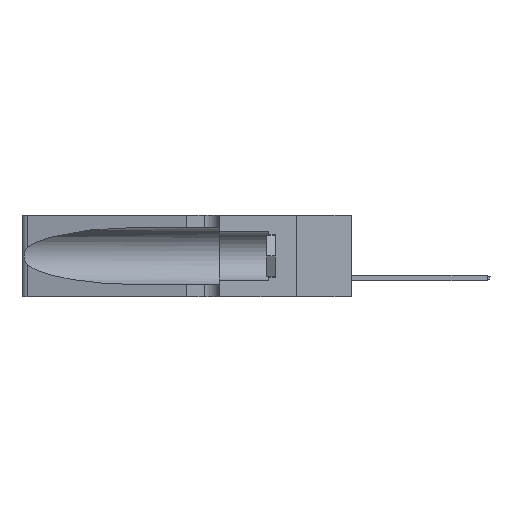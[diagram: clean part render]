
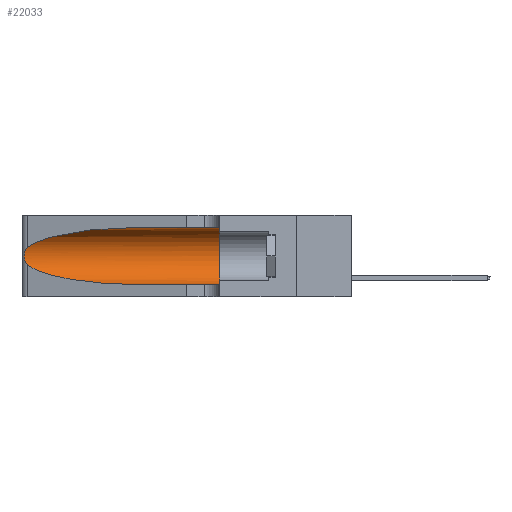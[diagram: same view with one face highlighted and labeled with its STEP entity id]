
A CAD part, left-side view. The second image highlights one B-rep face of the part: STEP entity #22033.
In plain terms, the highlighted cylindrical face has radius 3.308 mm (diameter 6.617 mm), a partial arc.
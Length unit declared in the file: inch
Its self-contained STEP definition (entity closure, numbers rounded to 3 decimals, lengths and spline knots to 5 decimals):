
#607 = LINE ( 'NONE', #9690, #24360 ) ;
#701 = AXIS2_PLACEMENT_3D ( 'NONE', #26707, #38250, #37762 ) ;
#719 = VERTEX_POINT ( 'NONE', #9431 ) ;
#1032 = CARTESIAN_POINT ( 'NONE',  ( 0.25487, 1.22718, 0.14631 ) ) ;
#1111 = CARTESIAN_POINT ( 'NONE',  ( 0.26075, 1.23896, 0.19203 ) ) ;
#1333 = EDGE_CURVE ( 'NONE', #11375, #21512, #15823, .T. ) ;
#2590 = ORIENTED_EDGE ( 'NONE', *, *, #46567, .F. ) ;
#2606 = FACE_OUTER_BOUND ( 'NONE', #6773, .T. ) ;
#3144 = CARTESIAN_POINT ( 'NONE',  ( 0.1305, 0.72297, 0.05475 ) ) ;
#4132 = DIRECTION ( 'NONE',  ( 0., -1., 0. ) ) ;
#6708 = CARTESIAN_POINT ( 'NONE',  ( 0.18966, 0.96281, 0.05475 ) ) ;
#6773 = EDGE_LOOP ( 'NONE', ( #46188, #41725, #33761, #12779, #41963, #2590 ) ) ;
#7079 = DIRECTION ( 'NONE',  ( 0., -1., 0. ) ) ;
#7232 =( BOUNDED_CURVE ( )  B_SPLINE_CURVE ( 3, ( #25480, #40543, #6708, #3144 ),
 .UNSPECIFIED., .F., .F. ) 
 B_SPLINE_CURVE_WITH_KNOTS ( ( 4, 4 ),
 ( 3.44316, 4.71239 ),
 .UNSPECIFIED. ) 
 CURVE ( )  GEOMETRIC_REPRESENTATION_ITEM ( )  RATIONAL_B_SPLINE_CURVE ( ( 1., 0.87, 0.87, 1. ) ) 
 REPRESENTATION_ITEM ( '' )  );
#8438 = CARTESIAN_POINT ( 'NONE',  ( 0.25487, 1.22718, 0.22369 ) ) ;
#9431 = CARTESIAN_POINT ( 'NONE',  ( 0.1305, 0.35, 0.05475 ) ) ;
#9690 = CARTESIAN_POINT ( 'NONE',  ( 0.1305, 1.61858, 0.31525 ) ) ;
#9915 = CARTESIAN_POINT ( 'NONE',  ( 0.18966, 0.96281, 0.31525 ) ) ;
#10462 = CARTESIAN_POINT ( 'NONE',  ( 0.25789, 1.23486, 0.15765 ) ) ;
#11375 = VERTEX_POINT ( 'NONE', #35086 ) ;
#11645 = CARTESIAN_POINT ( 'NONE',  ( 0.26018, 1.23835, 0.19895 ) ) ;
#12231 = CARTESIAN_POINT ( 'NONE',  ( 0.1305, 0.72297, 0.05475 ) ) ;
#12779 = ORIENTED_EDGE ( 'NONE', *, *, #28889, .T. ) ;
#14101 = CARTESIAN_POINT ( 'NONE',  ( 0.1305, 0.35, 0.31525 ) ) ;
#14140 = CARTESIAN_POINT ( 'NONE',  ( 0.25639, 1.23186, 0.15144 ) ) ;
#14295 = CARTESIAN_POINT ( 'NONE',  ( 0.25856, 1.23593, 0.16098 ) ) ;
#14339 = B_SPLINE_CURVE_WITH_KNOTS ( 'NONE', 3,
 ( #8438, #29938, #14866, #33815, #18904, #11645, #1111, #27666, #47364, #14295, #10462, #14140, #43826, #21589 ),
 .UNSPECIFIED., .F., .F.,
 ( 4, 2, 2, 2, 2, 2, 4 ),
 ( 0., 0.00027, 0.00053, 0.00107, 0.0016, 0.00187, 0.00214 ),
 .UNSPECIFIED. ) ;
#14866 = CARTESIAN_POINT ( 'NONE',  ( 0.25639, 1.23184, 0.21858 ) ) ;
#15823 =( BOUNDED_CURVE ( )  B_SPLINE_CURVE ( 3, ( #32059, #9915, #36170, #21536 ),
 .UNSPECIFIED., .F., .T. ) 
 B_SPLINE_CURVE_WITH_KNOTS ( ( 4, 4 ),
 ( 1.5708, 2.84003 ),
 .UNSPECIFIED. ) 
 CURVE ( )  GEOMETRIC_REPRESENTATION_ITEM ( )  RATIONAL_B_SPLINE_CURVE ( ( 1., 0.87, 0.87, 1. ) ) 
 REPRESENTATION_ITEM ( '' )  );
#16710 = VERTEX_POINT ( 'NONE', #12231 ) ;
#18904 = CARTESIAN_POINT ( 'NONE',  ( 0.25854, 1.2359, 0.20912 ) ) ;
#19135 = CARTESIAN_POINT ( 'NONE',  ( 0.1305, 1.61858, 0.05475 ) ) ;
#19322 = EDGE_CURVE ( 'NONE', #21512, #39578, #14339, .T. ) ;
#19472 = CARTESIAN_POINT ( 'NONE',  ( 0.1305, 0.35, 0.185 ) ) ;
#20396 = EDGE_CURVE ( 'NONE', #39578, #16710, #7232, .T. ) ;
#21512 = VERTEX_POINT ( 'NONE', #35257 ) ;
#21536 = CARTESIAN_POINT ( 'NONE',  ( 0.25487, 1.22718, 0.22369 ) ) ;
#21589 = CARTESIAN_POINT ( 'NONE',  ( 0.25487, 1.22718, 0.14631 ) ) ;
#22033 = ADVANCED_FACE ( 'NONE', ( #2606 ), #30418, .F. ) ;
#23859 = DIRECTION ( 'NONE',  ( 0., 1., 0. ) ) ;
#24360 = VECTOR ( 'NONE', #7079, 39.37008 ) ;
#25480 = CARTESIAN_POINT ( 'NONE',  ( 0.25487, 1.22718, 0.14631 ) ) ;
#26707 = CARTESIAN_POINT ( 'NONE',  ( 0.1305, 1.61858, 0.185 ) ) ;
#27506 = CIRCLE ( 'NONE', #36412, 0.13025 ) ;
#27666 = CARTESIAN_POINT ( 'NONE',  ( 0.26075, 1.23896, 0.178 ) ) ;
#28889 = EDGE_CURVE ( 'NONE', #16710, #719, #42220, .T. ) ;
#29938 = CARTESIAN_POINT ( 'NONE',  ( 0.25555, 1.22994, 0.2215 ) ) ;
#30418 = CYLINDRICAL_SURFACE ( 'NONE', #701, 0.13025 ) ;
#30757 = EDGE_CURVE ( 'NONE', #40463, #719, #27506, .T. ) ;
#32059 = CARTESIAN_POINT ( 'NONE',  ( 0.1305, 0.72297, 0.31525 ) ) ;
#32318 = VECTOR ( 'NONE', #4132, 39.37008 ) ;
#33761 = ORIENTED_EDGE ( 'NONE', *, *, #20396, .T. ) ;
#33815 = CARTESIAN_POINT ( 'NONE',  ( 0.25787, 1.23484, 0.2124 ) ) ;
#35086 = CARTESIAN_POINT ( 'NONE',  ( 0.1305, 0.72297, 0.31525 ) ) ;
#35257 = CARTESIAN_POINT ( 'NONE',  ( 0.25487, 1.22718, 0.22369 ) ) ;
#36170 = CARTESIAN_POINT ( 'NONE',  ( 0.2373, 1.15595, 0.28018 ) ) ;
#36412 = AXIS2_PLACEMENT_3D ( 'NONE', #19472, #23859, #41895 ) ;
#37762 = DIRECTION ( 'NONE',  ( 0., 0., -1. ) ) ;
#38250 = DIRECTION ( 'NONE',  ( 0., -1., 0. ) ) ;
#39578 = VERTEX_POINT ( 'NONE', #1032 ) ;
#40463 = VERTEX_POINT ( 'NONE', #14101 ) ;
#40543 = CARTESIAN_POINT ( 'NONE',  ( 0.2373, 1.15595, 0.08982 ) ) ;
#41725 = ORIENTED_EDGE ( 'NONE', *, *, #19322, .T. ) ;
#41895 = DIRECTION ( 'NONE',  ( 0., 0., 1. ) ) ;
#41963 = ORIENTED_EDGE ( 'NONE', *, *, #30757, .F. ) ;
#42220 = LINE ( 'NONE', #19135, #32318 ) ;
#43826 = CARTESIAN_POINT ( 'NONE',  ( 0.25555, 1.22993, 0.14849 ) ) ;
#46188 = ORIENTED_EDGE ( 'NONE', *, *, #1333, .T. ) ;
#46567 = EDGE_CURVE ( 'NONE', #11375, #40463, #607, .T. ) ;
#47364 = CARTESIAN_POINT ( 'NONE',  ( 0.26017, 1.23833, 0.17102 ) ) ;
